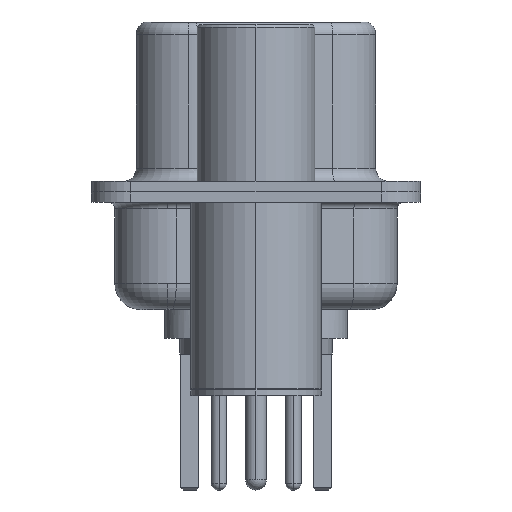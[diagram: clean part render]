
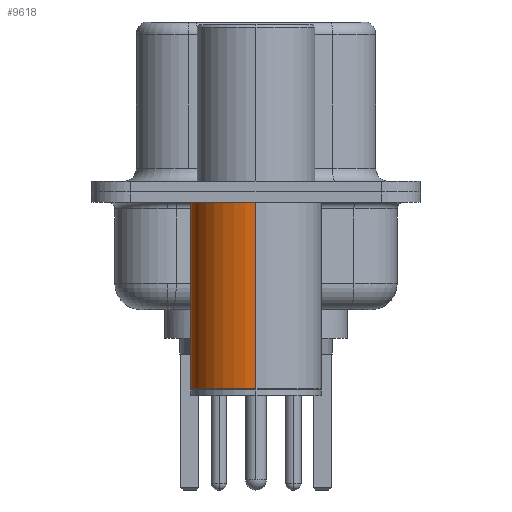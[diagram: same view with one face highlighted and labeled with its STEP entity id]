
A CAD part, left-side view. The second image highlights one B-rep face of the part: STEP entity #9618.
In plain terms, the highlighted cylindrical face has radius 2.5 mm (diameter 5 mm), a partial arc.
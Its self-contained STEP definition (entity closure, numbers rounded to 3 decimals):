
#342 = CARTESIAN_POINT ( 'NONE',  ( 2.5, 0., 0.581 ) ) ;
#2697 = ORIENTED_EDGE ( 'NONE', *, *, #9546, .T. ) ;
#3407 = DIRECTION ( 'NONE',  ( 1., 0., 0. ) ) ;
#3838 = FACE_OUTER_BOUND ( 'NONE', #23032, .T. ) ;
#4511 = DIRECTION ( 'NONE',  ( 0., 0., 1. ) ) ;
#5997 = CARTESIAN_POINT ( 'NONE',  ( 2.5, 0., -7.525 ) ) ;
#6504 = CARTESIAN_POINT ( 'NONE',  ( 0., 0., -0.4 ) ) ;
#6578 = ORIENTED_EDGE ( 'NONE', *, *, #9689, .F. ) ;
#6962 = VECTOR ( 'NONE', #9433, 1000. ) ;
#7513 = VERTEX_POINT ( 'NONE', #19901 ) ;
#8131 = CYLINDRICAL_SURFACE ( 'NONE', #22816, 2.5 ) ;
#8380 = DIRECTION ( 'NONE',  ( 1., 0., 0. ) ) ;
#8654 = CARTESIAN_POINT ( 'NONE',  ( -2.5, 0., 0.581 ) ) ;
#9433 = DIRECTION ( 'NONE',  ( 0., 0., 1. ) ) ;
#9546 = EDGE_CURVE ( 'NONE', #14240, #22243, #15378, .T. ) ;
#9618 = ADVANCED_FACE ( 'NONE', ( #3838 ), #8131, .T. ) ;
#9689 = EDGE_CURVE ( 'NONE', #15756, #7513, #21044, .T. ) ;
#9832 = EDGE_CURVE ( 'NONE', #15756, #14240, #14467, .T. ) ;
#10013 = EDGE_CURVE ( 'NONE', #7513, #22243, #10952, .T. ) ;
#10952 = CIRCLE ( 'NONE', #20714, 2.5 ) ;
#14240 = VERTEX_POINT ( 'NONE', #19873 ) ;
#14399 = DIRECTION ( 'NONE',  ( 0., 0., 1. ) ) ;
#14467 = CIRCLE ( 'NONE', #16331, 2.5 ) ;
#15378 = LINE ( 'NONE', #8654, #19656 ) ;
#15565 = CARTESIAN_POINT ( 'NONE',  ( 0., 0., -7.525 ) ) ;
#15756 = VERTEX_POINT ( 'NONE', #5997 ) ;
#16331 = AXIS2_PLACEMENT_3D ( 'NONE', #15565, #4511, #17437 ) ;
#17437 = DIRECTION ( 'NONE',  ( 1., 0., 0. ) ) ;
#18070 = CARTESIAN_POINT ( 'NONE',  ( 0., 0., 0.581 ) ) ;
#19422 = DIRECTION ( 'NONE',  ( 0., 0., 1. ) ) ;
#19656 = VECTOR ( 'NONE', #19720, 1000. ) ;
#19720 = DIRECTION ( 'NONE',  ( 0., 0., 1. ) ) ;
#19873 = CARTESIAN_POINT ( 'NONE',  ( -2.5, 0., -7.525 ) ) ;
#19901 = CARTESIAN_POINT ( 'NONE',  ( 2.5, 0., -0.4 ) ) ;
#20621 = ORIENTED_EDGE ( 'NONE', *, *, #10013, .F. ) ;
#20703 = ORIENTED_EDGE ( 'NONE', *, *, #9832, .T. ) ;
#20714 = AXIS2_PLACEMENT_3D ( 'NONE', #6504, #19422, #8380 ) ;
#21044 = LINE ( 'NONE', #342, #6962 ) ;
#21495 = CARTESIAN_POINT ( 'NONE',  ( -2.5, 0., -0.4 ) ) ;
#22243 = VERTEX_POINT ( 'NONE', #21495 ) ;
#22816 = AXIS2_PLACEMENT_3D ( 'NONE', #18070, #14399, #3407 ) ;
#23032 = EDGE_LOOP ( 'NONE', ( #20703, #2697, #20621, #6578 ) ) ;
